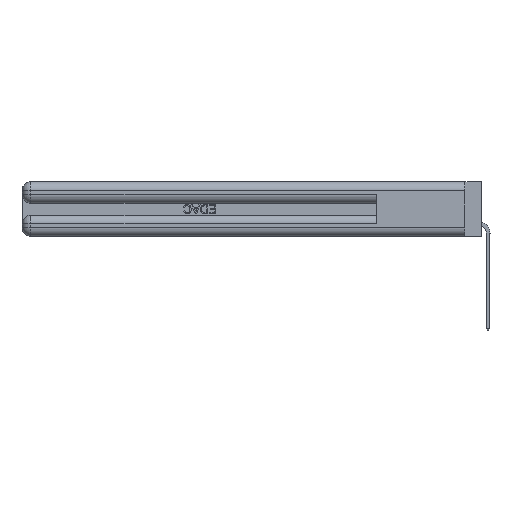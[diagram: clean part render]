
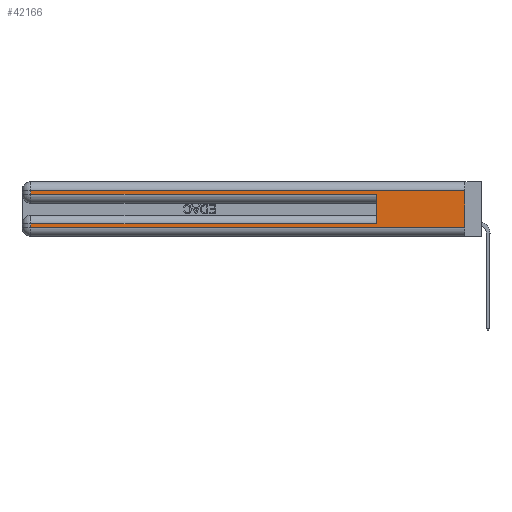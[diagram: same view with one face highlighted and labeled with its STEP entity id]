
A CAD part, left-side view. The second image highlights one B-rep face of the part: STEP entity #42166.
In plain terms, the highlighted planar face has unit normal (-1, 0, 0).
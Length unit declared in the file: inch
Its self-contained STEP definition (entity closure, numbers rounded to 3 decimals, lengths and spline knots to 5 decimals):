
#561 = CARTESIAN_POINT ( 'NONE',  ( 0., 0., 0.285 ) ) ;
#836 = LINE ( 'NONE', #5803, #15668 ) ;
#2070 = VERTEX_POINT ( 'NONE', #27128 ) ;
#2621 = EDGE_CURVE ( 'NONE', #34767, #43059, #29149, .T. ) ;
#3681 = CARTESIAN_POINT ( 'NONE',  ( 0., 0., 0.31 ) ) ;
#3917 = EDGE_CURVE ( 'NONE', #31295, #11055, #836, .T. ) ;
#4625 = CARTESIAN_POINT ( 'NONE',  ( 0., 0.6, 0.285 ) ) ;
#4799 = ORIENTED_EDGE ( 'NONE', *, *, #3917, .F. ) ;
#5782 = PLANE ( 'NONE',  #42388 ) ;
#5803 = CARTESIAN_POINT ( 'NONE',  ( 0., 0., 0.37 ) ) ;
#7090 = DIRECTION ( 'NONE',  ( 0., 0., -1. ) ) ;
#7616 = CARTESIAN_POINT ( 'NONE',  ( 0., 2.94, 0.37 ) ) ;
#8338 = DIRECTION ( 'NONE',  ( 0., 0., -1. ) ) ;
#8415 = EDGE_CURVE ( 'NONE', #2070, #15502, #14155, .T. ) ;
#8654 = CARTESIAN_POINT ( 'NONE',  ( 0., 0., 0.31 ) ) ;
#11055 = VERTEX_POINT ( 'NONE', #15746 ) ;
#11333 = DIRECTION ( 'NONE',  ( 0., 1., 0. ) ) ;
#12802 = DIRECTION ( 'NONE',  ( 0., 0., 1. ) ) ;
#13881 = ORIENTED_EDGE ( 'NONE', *, *, #39905, .T. ) ;
#13976 = LINE ( 'NONE', #3681, #30356 ) ;
#14155 = LINE ( 'NONE', #7616, #37909 ) ;
#15502 = VERTEX_POINT ( 'NONE', #28541 ) ;
#15607 = EDGE_CURVE ( 'NONE', #31295, #2070, #13976, .T. ) ;
#15668 = VECTOR ( 'NONE', #25071, 39.37008 ) ;
#15746 = CARTESIAN_POINT ( 'NONE',  ( 0., 0., 0.06 ) ) ;
#16233 = VERTEX_POINT ( 'NONE', #23533 ) ;
#16576 = EDGE_CURVE ( 'NONE', #34767, #40034, #23961, .T. ) ;
#17391 = ORIENTED_EDGE ( 'NONE', *, *, #15607, .T. ) ;
#19747 = VECTOR ( 'NONE', #11333, 39.37008 ) ;
#20508 = DIRECTION ( 'NONE',  ( 0., 0., -1. ) ) ;
#20873 = VECTOR ( 'NONE', #7090, 39.37008 ) ;
#22403 = ORIENTED_EDGE ( 'NONE', *, *, #16576, .T. ) ;
#23533 = CARTESIAN_POINT ( 'NONE',  ( 0., 2.94, 0.06 ) ) ;
#23582 = EDGE_CURVE ( 'NONE', #16233, #11055, #30596, .T. ) ;
#23961 = LINE ( 'NONE', #34479, #19747 ) ;
#24714 = ORIENTED_EDGE ( 'NONE', *, *, #39031, .T. ) ;
#25071 = DIRECTION ( 'NONE',  ( 0., 0., -1. ) ) ;
#26565 = ORIENTED_EDGE ( 'NONE', *, *, #23582, .T. ) ;
#26719 = LINE ( 'NONE', #27319, #20873 ) ;
#27128 = CARTESIAN_POINT ( 'NONE',  ( 0., 2.94, 0.31 ) ) ;
#27319 = CARTESIAN_POINT ( 'NONE',  ( 0., 2.94, 0.37 ) ) ;
#28278 = ORIENTED_EDGE ( 'NONE', *, *, #2621, .F. ) ;
#28451 = VECTOR ( 'NONE', #30643, 39.37008 ) ;
#28541 = CARTESIAN_POINT ( 'NONE',  ( 0., 2.94, 0.285 ) ) ;
#29149 = LINE ( 'NONE', #36246, #42967 ) ;
#30356 = VECTOR ( 'NONE', #38486, 39.37008 ) ;
#30596 = LINE ( 'NONE', #37448, #28451 ) ;
#30643 = DIRECTION ( 'NONE',  ( 0., -1., 0. ) ) ;
#31295 = VERTEX_POINT ( 'NONE', #8654 ) ;
#31580 = CARTESIAN_POINT ( 'NONE',  ( 0., 2.94, 0.085 ) ) ;
#32514 = EDGE_LOOP ( 'NONE', ( #4799, #17391, #33239, #13881, #28278, #22403, #24714, #26565 ) ) ;
#32753 = DIRECTION ( 'NONE',  ( 1., 0., 0. ) ) ;
#33239 = ORIENTED_EDGE ( 'NONE', *, *, #8415, .T. ) ;
#34372 = DIRECTION ( 'NONE',  ( 0., -1., 0. ) ) ;
#34441 = CARTESIAN_POINT ( 'NONE',  ( 0., 0.6, 0.085 ) ) ;
#34479 = CARTESIAN_POINT ( 'NONE',  ( 0., 0., 0.085 ) ) ;
#34767 = VERTEX_POINT ( 'NONE', #34441 ) ;
#36133 = LINE ( 'NONE', #561, #39317 ) ;
#36246 = CARTESIAN_POINT ( 'NONE',  ( 0., 0.6, 0.145 ) ) ;
#37448 = CARTESIAN_POINT ( 'NONE',  ( 0., 0., 0.06 ) ) ;
#37909 = VECTOR ( 'NONE', #8338, 39.37008 ) ;
#38486 = DIRECTION ( 'NONE',  ( 0., 1., 0. ) ) ;
#38634 = FACE_OUTER_BOUND ( 'NONE', #32514, .T. ) ;
#39031 = EDGE_CURVE ( 'NONE', #40034, #16233, #26719, .T. ) ;
#39317 = VECTOR ( 'NONE', #34372, 39.37008 ) ;
#39752 = CARTESIAN_POINT ( 'NONE',  ( 0., 0., 0.37 ) ) ;
#39905 = EDGE_CURVE ( 'NONE', #15502, #43059, #36133, .T. ) ;
#40034 = VERTEX_POINT ( 'NONE', #31580 ) ;
#42166 = ADVANCED_FACE ( 'NONE', ( #38634 ), #5782, .F. ) ;
#42388 = AXIS2_PLACEMENT_3D ( 'NONE', #39752, #32753, #20508 ) ;
#42967 = VECTOR ( 'NONE', #12802, 39.37008 ) ;
#43059 = VERTEX_POINT ( 'NONE', #4625 ) ;
